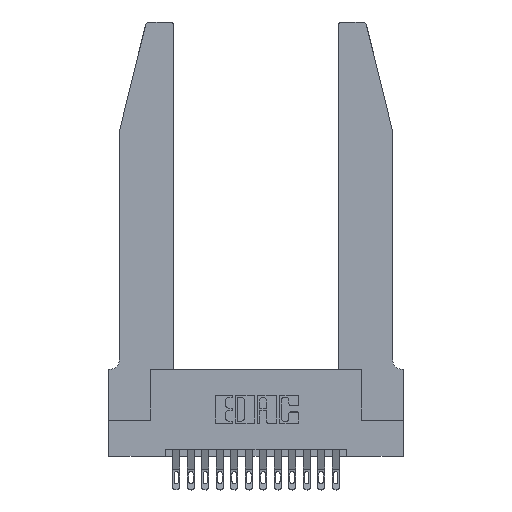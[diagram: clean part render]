
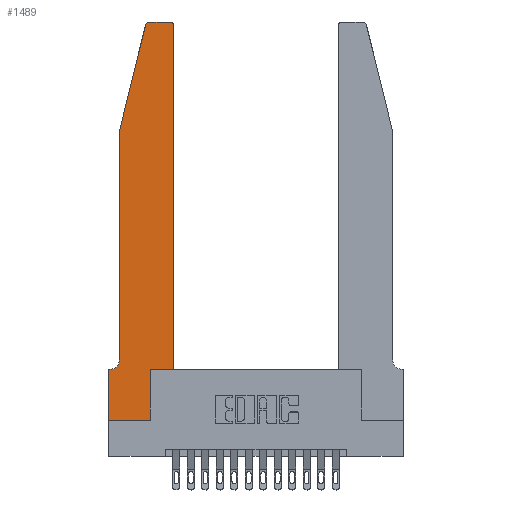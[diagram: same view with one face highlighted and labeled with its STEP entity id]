
A CAD part, top view. The second image highlights one B-rep face of the part: STEP entity #1489.
In plain terms, the highlighted planar face has unit normal (0, 0, 1).
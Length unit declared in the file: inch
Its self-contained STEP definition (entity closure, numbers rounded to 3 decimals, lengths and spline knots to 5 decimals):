
#127 = VECTOR ( 'NONE', #18176, 39.37008 ) ;
#386 = CARTESIAN_POINT ( 'NONE',  ( 0., 0.35, 0.37 ) ) ;
#448 = DIRECTION ( 'NONE',  ( 0., 0., 1. ) ) ;
#501 = VERTEX_POINT ( 'NONE', #12518 ) ;
#766 = CARTESIAN_POINT ( 'NONE',  ( 0., 0.35, 0.37 ) ) ;
#850 = FACE_OUTER_BOUND ( 'NONE', #8025, .T. ) ;
#901 = LINE ( 'NONE', #4100, #4706 ) ;
#930 = VECTOR ( 'NONE', #12539, 39.37008 ) ;
#1323 = CARTESIAN_POINT ( 'NONE',  ( 0.0755, 0.42, 0.37 ) ) ;
#1489 = ADVANCED_FACE ( 'NONE', ( #850 ), #7370, .T. ) ;
#2228 = VECTOR ( 'NONE', #13955, 39.37008 ) ;
#2277 = VECTOR ( 'NONE', #14926, 39.37008 ) ;
#2309 = AXIS2_PLACEMENT_3D ( 'NONE', #9528, #3585, #18200 ) ;
#2536 = CARTESIAN_POINT ( 'NONE',  ( 0.2865, 0.35, 0.37 ) ) ;
#2558 = ORIENTED_EDGE ( 'NONE', *, *, #5326, .T. ) ;
#2559 = CARTESIAN_POINT ( 'NONE',  ( 0.0755, 0.35, 0.37 ) ) ;
#2574 = CARTESIAN_POINT ( 'NONE',  ( 0., 0., 0.37 ) ) ;
#2746 = LINE ( 'NONE', #12026, #2277 ) ;
#2956 = EDGE_CURVE ( 'NONE', #7157, #16706, #5729, .T. ) ;
#3403 = CARTESIAN_POINT ( 'NONE',  ( 0.25487, 2.72718, 0.37 ) ) ;
#3585 = DIRECTION ( 'NONE',  ( 0., 0., -1. ) ) ;
#3612 = EDGE_CURVE ( 'NONE', #501, #13807, #9721, .T. ) ;
#3835 = ORIENTED_EDGE ( 'NONE', *, *, #13346, .T. ) ;
#4091 = ORIENTED_EDGE ( 'NONE', *, *, #11307, .T. ) ;
#4100 = CARTESIAN_POINT ( 'NONE',  ( 0.2605, 2.75, 0.37 ) ) ;
#4498 = VERTEX_POINT ( 'NONE', #5972 ) ;
#4706 = VECTOR ( 'NONE', #5606, 39.37008 ) ;
#4779 = CARTESIAN_POINT ( 'NONE',  ( 0.0755, 2., 0.37 ) ) ;
#4838 = CIRCLE ( 'NONE', #17151, 0.03 ) ;
#5326 = EDGE_CURVE ( 'NONE', #14672, #7157, #16483, .T. ) ;
#5414 = DIRECTION ( 'NONE',  ( 0., -1., 0. ) ) ;
#5593 = VERTEX_POINT ( 'NONE', #5803 ) ;
#5606 = DIRECTION ( 'NONE',  ( -1., 0., 0. ) ) ;
#5729 = CIRCLE ( 'NONE', #2309, 0.07 ) ;
#5803 = CARTESIAN_POINT ( 'NONE',  ( 0.284, 2.75, 0.37 ) ) ;
#5972 = CARTESIAN_POINT ( 'NONE',  ( 0.2865, 0., 0.37 ) ) ;
#6257 = EDGE_CURVE ( 'NONE', #4498, #6614, #18496, .T. ) ;
#6378 = VECTOR ( 'NONE', #5414, 39.37008 ) ;
#6614 = VERTEX_POINT ( 'NONE', #2536 ) ;
#7157 = VERTEX_POINT ( 'NONE', #1323 ) ;
#7370 = PLANE ( 'NONE',  #13301 ) ;
#7374 = ORIENTED_EDGE ( 'NONE', *, *, #9077, .T. ) ;
#7478 = EDGE_CURVE ( 'NONE', #6614, #501, #12591, .T. ) ;
#7601 = ORIENTED_EDGE ( 'NONE', *, *, #2956, .T. ) ;
#7717 = CARTESIAN_POINT ( 'NONE',  ( 0.0055, 0.35, 0.37 ) ) ;
#7893 = CARTESIAN_POINT ( 'NONE',  ( 0.4505, 2.72, 0.37 ) ) ;
#7999 = ORIENTED_EDGE ( 'NONE', *, *, #14992, .T. ) ;
#8025 = EDGE_LOOP ( 'NONE', ( #13695, #3835, #11647, #2558, #7601, #7999, #7374, #9788, #18554, #12561, #15569, #4091 ) ) ;
#8168 = CARTESIAN_POINT ( 'NONE',  ( 0.0755, 2., 0.37 ) ) ;
#8683 = EDGE_CURVE ( 'NONE', #14957, #4498, #15272, .T. ) ;
#9077 = EDGE_CURVE ( 'NONE', #17718, #14957, #2746, .T. ) ;
#9309 = CARTESIAN_POINT ( 'NONE',  ( 0.4505, 0.35, 0.37 ) ) ;
#9528 = CARTESIAN_POINT ( 'NONE',  ( 0.0055, 0.42, 0.37 ) ) ;
#9721 = LINE ( 'NONE', #9309, #127 ) ;
#9750 = DIRECTION ( 'NONE',  ( 0., 1., 0. ) ) ;
#9788 = ORIENTED_EDGE ( 'NONE', *, *, #8683, .T. ) ;
#10191 = DIRECTION ( 'NONE',  ( -0.239, -0.971, 0. ) ) ;
#10370 = CARTESIAN_POINT ( 'NONE',  ( 0.4205, 2.75, 0.37 ) ) ;
#10432 = CARTESIAN_POINT ( 'NONE',  ( 0.0755, 2., 0.37 ) ) ;
#10837 = VERTEX_POINT ( 'NONE', #3403 ) ;
#11015 = CIRCLE ( 'NONE', #17184, 0.03 ) ;
#11307 = EDGE_CURVE ( 'NONE', #13807, #13496, #4838, .T. ) ;
#11357 = DIRECTION ( 'NONE',  ( 0., 0., 1. ) ) ;
#11471 = DIRECTION ( 'NONE',  ( 0., 0., 1. ) ) ;
#11477 = EDGE_CURVE ( 'NONE', #10837, #14672, #15616, .T. ) ;
#11647 = ORIENTED_EDGE ( 'NONE', *, *, #11477, .T. ) ;
#12026 = CARTESIAN_POINT ( 'NONE',  ( 0., 0., 0.37 ) ) ;
#12242 = LINE ( 'NONE', #2559, #2228 ) ;
#12518 = CARTESIAN_POINT ( 'NONE',  ( 0.4505, 0.35, 0.37 ) ) ;
#12539 = DIRECTION ( 'NONE',  ( 1., 0., 0. ) ) ;
#12561 = ORIENTED_EDGE ( 'NONE', *, *, #7478, .T. ) ;
#12591 = LINE ( 'NONE', #18447, #16639 ) ;
#12739 = DIRECTION ( 'NONE',  ( 1., 0., 0. ) ) ;
#13301 = AXIS2_PLACEMENT_3D ( 'NONE', #386, #448, #16165 ) ;
#13346 = EDGE_CURVE ( 'NONE', #5593, #10837, #11015, .T. ) ;
#13496 = VERTEX_POINT ( 'NONE', #10370 ) ;
#13695 = ORIENTED_EDGE ( 'NONE', *, *, #17059, .T. ) ;
#13807 = VERTEX_POINT ( 'NONE', #7893 ) ;
#13955 = DIRECTION ( 'NONE',  ( -1., 0., 0. ) ) ;
#14450 = VECTOR ( 'NONE', #9750, 39.37008 ) ;
#14672 = VERTEX_POINT ( 'NONE', #4779 ) ;
#14926 = DIRECTION ( 'NONE',  ( 0., -1., 0. ) ) ;
#14957 = VERTEX_POINT ( 'NONE', #15565 ) ;
#14992 = EDGE_CURVE ( 'NONE', #16706, #17718, #12242, .T. ) ;
#15272 = LINE ( 'NONE', #2574, #930 ) ;
#15565 = CARTESIAN_POINT ( 'NONE',  ( 0., 0., 0.37 ) ) ;
#15569 = ORIENTED_EDGE ( 'NONE', *, *, #3612, .T. ) ;
#15581 = CARTESIAN_POINT ( 'NONE',  ( 0.4205, 2.72, 0.37 ) ) ;
#15616 = LINE ( 'NONE', #10432, #17855 ) ;
#15912 = CARTESIAN_POINT ( 'NONE',  ( 0.284, 2.72, 0.37 ) ) ;
#16165 = DIRECTION ( 'NONE',  ( 1., 0., 0. ) ) ;
#16306 = DIRECTION ( 'NONE',  ( 1., 0., 0. ) ) ;
#16483 = LINE ( 'NONE', #8168, #6378 ) ;
#16639 = VECTOR ( 'NONE', #16876, 39.37008 ) ;
#16706 = VERTEX_POINT ( 'NONE', #7717 ) ;
#16876 = DIRECTION ( 'NONE',  ( 1., 0., 0. ) ) ;
#17059 = EDGE_CURVE ( 'NONE', #13496, #5593, #901, .T. ) ;
#17151 = AXIS2_PLACEMENT_3D ( 'NONE', #15581, #11471, #16306 ) ;
#17184 = AXIS2_PLACEMENT_3D ( 'NONE', #15912, #11357, #12739 ) ;
#17718 = VERTEX_POINT ( 'NONE', #766 ) ;
#17855 = VECTOR ( 'NONE', #10191, 39.37008 ) ;
#18176 = DIRECTION ( 'NONE',  ( 0., 1., 0. ) ) ;
#18200 = DIRECTION ( 'NONE',  ( -1., 0., 0. ) ) ;
#18361 = CARTESIAN_POINT ( 'NONE',  ( 0.2865, 0.35, 0.37 ) ) ;
#18447 = CARTESIAN_POINT ( 'NONE',  ( 0.4505, 0.35, 0.37 ) ) ;
#18496 = LINE ( 'NONE', #18361, #14450 ) ;
#18554 = ORIENTED_EDGE ( 'NONE', *, *, #6257, .T. ) ;
